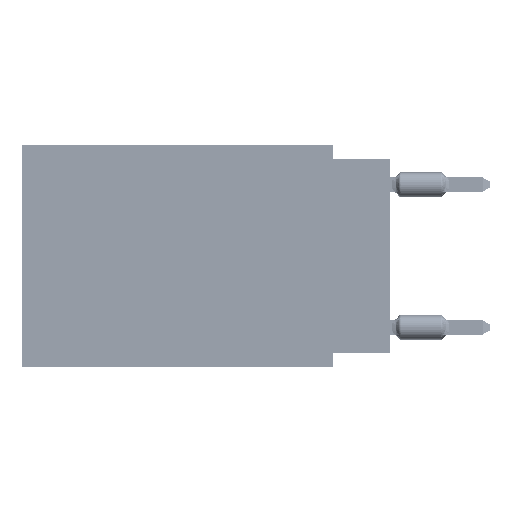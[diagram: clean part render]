
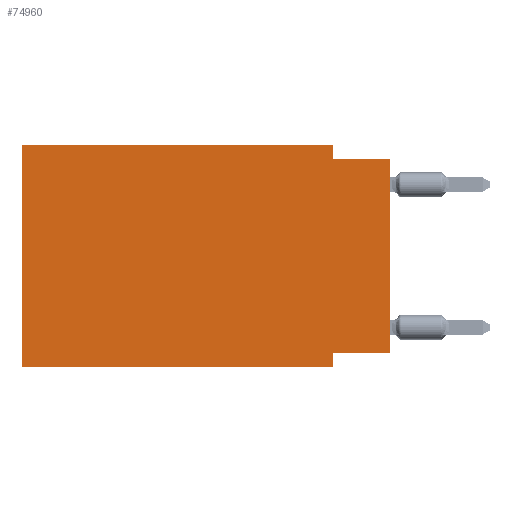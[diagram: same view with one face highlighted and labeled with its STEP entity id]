
A CAD part, left-side view. The second image highlights one B-rep face of the part: STEP entity #74960.
In plain terms, the highlighted planar face has unit normal (-1, 0, 0).
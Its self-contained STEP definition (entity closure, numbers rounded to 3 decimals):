
#1953 = FACE_OUTER_BOUND ( 'NONE', #66279, .T. ) ;
#2069 = DIRECTION ( 'NONE',  ( 0., 0., -1. ) ) ;
#2941 = LINE ( 'NONE', #45342, #27557 ) ;
#3453 = EDGE_CURVE ( 'NONE', #26817, #6976, #25325, .T. ) ;
#3585 = AXIS2_PLACEMENT_3D ( 'NONE', #43198, #7836, #7062 ) ;
#4866 = CARTESIAN_POINT ( 'NONE',  ( 0., 0., 0. ) ) ;
#6976 = VERTEX_POINT ( 'NONE', #39225 ) ;
#7062 = DIRECTION ( 'NONE',  ( 0., 0., -1. ) ) ;
#7836 = DIRECTION ( 'NONE',  ( 1., 0., 0. ) ) ;
#15681 = ORIENTED_EDGE ( 'NONE', *, *, #67957, .F. ) ;
#18301 = ORIENTED_EDGE ( 'NONE', *, *, #20804, .F. ) ;
#18342 = VERTEX_POINT ( 'NONE', #73987 ) ;
#18770 = CARTESIAN_POINT ( 'NONE',  ( 0., 0., -0.635 ) ) ;
#19090 = VECTOR ( 'NONE', #67020, 1000. ) ;
#19320 = CARTESIAN_POINT ( 'NONE',  ( 0., 0., -0.635 ) ) ;
#20168 = LINE ( 'NONE', #67734, #51973 ) ;
#20701 = CARTESIAN_POINT ( 'NONE',  ( 0., 16.383, -9.906 ) ) ;
#20804 = EDGE_CURVE ( 'NONE', #6976, #57852, #20168, .T. ) ;
#21092 = EDGE_CURVE ( 'NONE', #51808, #51480, #77479, .T. ) ;
#25325 = LINE ( 'NONE', #37517, #19090 ) ;
#25869 = ORIENTED_EDGE ( 'NONE', *, *, #33398, .T. ) ;
#25871 = PLANE ( 'NONE',  #3585 ) ;
#26817 = VERTEX_POINT ( 'NONE', #37001 ) ;
#27557 = VECTOR ( 'NONE', #33934, 1000. ) ;
#28696 = VECTOR ( 'NONE', #56859, 1000. ) ;
#31964 = DIRECTION ( 'NONE',  ( 0., -1., 0. ) ) ;
#33173 = CARTESIAN_POINT ( 'NONE',  ( 0., 2.54, -9.906 ) ) ;
#33398 = EDGE_CURVE ( 'NONE', #26817, #36144, #38021, .T. ) ;
#33934 = DIRECTION ( 'NONE',  ( 0., 0., -1. ) ) ;
#34323 = EDGE_CURVE ( 'NONE', #57852, #18342, #2941, .T. ) ;
#35759 = VECTOR ( 'NONE', #58691, 1000. ) ;
#36144 = VERTEX_POINT ( 'NONE', #33173 ) ;
#37001 = CARTESIAN_POINT ( 'NONE',  ( 0., 16.383, -9.906 ) ) ;
#37517 = CARTESIAN_POINT ( 'NONE',  ( 0., 16.383, 0. ) ) ;
#38021 = LINE ( 'NONE', #20701, #28696 ) ;
#39225 = CARTESIAN_POINT ( 'NONE',  ( 0., 16.383, 0. ) ) ;
#41752 = CARTESIAN_POINT ( 'NONE',  ( 0., 0., -9.271 ) ) ;
#41981 = CARTESIAN_POINT ( 'NONE',  ( 0., 2.54, 0. ) ) ;
#42840 = ORIENTED_EDGE ( 'NONE', *, *, #69284, .F. ) ;
#43198 = CARTESIAN_POINT ( 'NONE',  ( 0., 16.383, 0. ) ) ;
#45342 = CARTESIAN_POINT ( 'NONE',  ( 0., 2.54, 0. ) ) ;
#47990 = VECTOR ( 'NONE', #2069, 1000. ) ;
#48018 = DIRECTION ( 'NONE',  ( 0., 1., 0. ) ) ;
#51480 = VERTEX_POINT ( 'NONE', #55317 ) ;
#51808 = VERTEX_POINT ( 'NONE', #67032 ) ;
#51973 = VECTOR ( 'NONE', #31964, 1000. ) ;
#53824 = ORIENTED_EDGE ( 'NONE', *, *, #3453, .F. ) ;
#54340 = LINE ( 'NONE', #55879, #47990 ) ;
#54486 = VERTEX_POINT ( 'NONE', #18770 ) ;
#54922 = ORIENTED_EDGE ( 'NONE', *, *, #21092, .F. ) ;
#55317 = CARTESIAN_POINT ( 'NONE',  ( 0., 2.54, -9.271 ) ) ;
#55879 = CARTESIAN_POINT ( 'NONE',  ( 0., 2.54, -9.906 ) ) ;
#56859 = DIRECTION ( 'NONE',  ( 0., -1., 0. ) ) ;
#57852 = VERTEX_POINT ( 'NONE', #41981 ) ;
#57983 = ORIENTED_EDGE ( 'NONE', *, *, #34323, .F. ) ;
#58691 = DIRECTION ( 'NONE',  ( 0., 0., 1. ) ) ;
#60867 = VECTOR ( 'NONE', #48018, 1000. ) ;
#65382 = LINE ( 'NONE', #4866, #35759 ) ;
#66279 = EDGE_LOOP ( 'NONE', ( #70294, #15681, #57983, #18301, #53824, #25869, #42840, #54922 ) ) ;
#67020 = DIRECTION ( 'NONE',  ( 0., 0., 1. ) ) ;
#67032 = CARTESIAN_POINT ( 'NONE',  ( 0., 0., -9.271 ) ) ;
#67278 = DIRECTION ( 'NONE',  ( 0., -1., 0. ) ) ;
#67734 = CARTESIAN_POINT ( 'NONE',  ( 0., 16.383, 0. ) ) ;
#67957 = EDGE_CURVE ( 'NONE', #18342, #54486, #73179, .T. ) ;
#69284 = EDGE_CURVE ( 'NONE', #51480, #36144, #54340, .T. ) ;
#70294 = ORIENTED_EDGE ( 'NONE', *, *, #72186, .T. ) ;
#70736 = VECTOR ( 'NONE', #67278, 1000. ) ;
#72186 = EDGE_CURVE ( 'NONE', #51808, #54486, #65382, .T. ) ;
#73179 = LINE ( 'NONE', #19320, #70736 ) ;
#73987 = CARTESIAN_POINT ( 'NONE',  ( 0., 2.54, -0.635 ) ) ;
#74960 = ADVANCED_FACE ( 'NONE', ( #1953 ), #25871, .F. ) ;
#77479 = LINE ( 'NONE', #41752, #60867 ) ;
